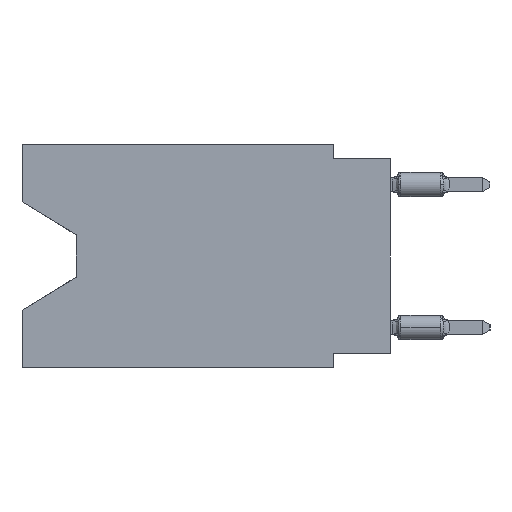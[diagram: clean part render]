
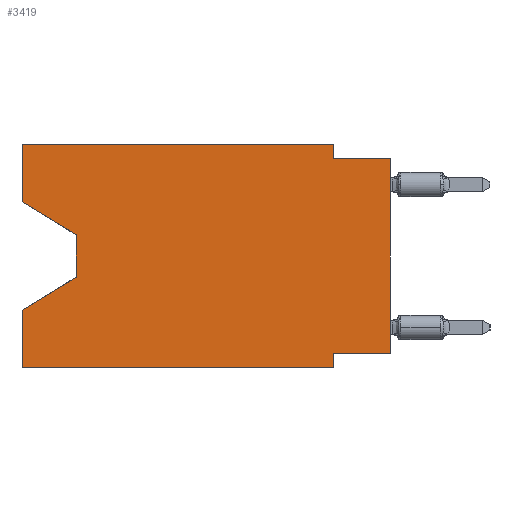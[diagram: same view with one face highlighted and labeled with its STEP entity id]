
A CAD part, left-side view. The second image highlights one B-rep face of the part: STEP entity #3419.
In plain terms, the highlighted planar face has unit normal (-1, 0, 0).
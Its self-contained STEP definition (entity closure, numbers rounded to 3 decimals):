
#75 = CARTESIAN_POINT ( 'NONE',  ( 0., 16.383, 0. ) ) ;
#409 = VERTEX_POINT ( 'NONE', #22014 ) ;
#544 = LINE ( 'NONE', #12322, #35364 ) ;
#1383 = DIRECTION ( 'NONE',  ( 0., -0.855, -0.519 ) ) ;
#1405 = ORIENTED_EDGE ( 'NONE', *, *, #28028, .F. ) ;
#1562 = DIRECTION ( 'NONE',  ( 0., 0., -1. ) ) ;
#2207 = DIRECTION ( 'NONE',  ( 0., 0.855, -0.519 ) ) ;
#2559 = VECTOR ( 'NONE', #2207, 1000. ) ;
#2894 = DIRECTION ( 'NONE',  ( 0., 0., -1. ) ) ;
#3386 = CARTESIAN_POINT ( 'NONE',  ( 0., 0., -9.271 ) ) ;
#3419 = ADVANCED_FACE ( 'NONE', ( #14137 ), #25959, .F. ) ;
#3909 = VERTEX_POINT ( 'NONE', #11076 ) ;
#5049 = EDGE_CURVE ( 'NONE', #409, #8129, #7990, .T. ) ;
#5308 = CARTESIAN_POINT ( 'NONE',  ( 0., 13.97, -5.893 ) ) ;
#6658 = CARTESIAN_POINT ( 'NONE',  ( 0., 16.383, -9.906 ) ) ;
#6813 = LINE ( 'NONE', #12984, #12689 ) ;
#7550 = CARTESIAN_POINT ( 'NONE',  ( 0., 2.54, -0.635 ) ) ;
#7679 = CARTESIAN_POINT ( 'NONE',  ( 0., 16.383, -2.546 ) ) ;
#7990 = LINE ( 'NONE', #5308, #2559 ) ;
#8129 = VERTEX_POINT ( 'NONE', #30926 ) ;
#8517 = EDGE_CURVE ( 'NONE', #10691, #29072, #544, .T. ) ;
#8570 = LINE ( 'NONE', #75, #35928 ) ;
#8912 = DIRECTION ( 'NONE',  ( 1., 0., 0. ) ) ;
#9150 = DIRECTION ( 'NONE',  ( 0., 0., 1. ) ) ;
#9357 = DIRECTION ( 'NONE',  ( 0., 1., 0. ) ) ;
#9603 = VECTOR ( 'NONE', #15794, 1000. ) ;
#9786 = VECTOR ( 'NONE', #32987, 1000. ) ;
#10060 = ORIENTED_EDGE ( 'NONE', *, *, #29583, .T. ) ;
#10117 = VECTOR ( 'NONE', #2894, 1000. ) ;
#10691 = VERTEX_POINT ( 'NONE', #7550 ) ;
#11076 = CARTESIAN_POINT ( 'NONE',  ( 0., 2.54, -9.271 ) ) ;
#12077 = LINE ( 'NONE', #3386, #18092 ) ;
#12322 = CARTESIAN_POINT ( 'NONE',  ( 0., 0., -0.635 ) ) ;
#12349 = CARTESIAN_POINT ( 'NONE',  ( 0., 16.383, 0. ) ) ;
#12626 = EDGE_CURVE ( 'NONE', #19016, #3909, #12077, .T. ) ;
#12689 = VECTOR ( 'NONE', #1383, 1000. ) ;
#12698 = LINE ( 'NONE', #18308, #9603 ) ;
#12715 = EDGE_CURVE ( 'NONE', #28179, #22189, #30252, .T. ) ;
#12984 = CARTESIAN_POINT ( 'NONE',  ( 0., 16.383, -2.546 ) ) ;
#13212 = ORIENTED_EDGE ( 'NONE', *, *, #19377, .T. ) ;
#14137 = FACE_OUTER_BOUND ( 'NONE', #32983, .T. ) ;
#14534 = ORIENTED_EDGE ( 'NONE', *, *, #25354, .F. ) ;
#14925 = LINE ( 'NONE', #23454, #29305 ) ;
#15179 = DIRECTION ( 'NONE',  ( 0., 0., 1. ) ) ;
#15706 = VECTOR ( 'NONE', #21638, 1000. ) ;
#15775 = CARTESIAN_POINT ( 'NONE',  ( 0., 16.383, -9.906 ) ) ;
#15794 = DIRECTION ( 'NONE',  ( 0., 0., 1. ) ) ;
#16940 = ORIENTED_EDGE ( 'NONE', *, *, #20787, .T. ) ;
#17511 = EDGE_CURVE ( 'NONE', #36996, #10691, #26676, .T. ) ;
#18067 = CARTESIAN_POINT ( 'NONE',  ( 0., 16.383, 0. ) ) ;
#18092 = VECTOR ( 'NONE', #9357, 1000. ) ;
#18308 = CARTESIAN_POINT ( 'NONE',  ( 0., 0., 0. ) ) ;
#18381 = EDGE_CURVE ( 'NONE', #3909, #23698, #22638, .T. ) ;
#19016 = VERTEX_POINT ( 'NONE', #21206 ) ;
#19377 = EDGE_CURVE ( 'NONE', #23972, #409, #14925, .T. ) ;
#20613 = ORIENTED_EDGE ( 'NONE', *, *, #12626, .F. ) ;
#20787 = EDGE_CURVE ( 'NONE', #28179, #23972, #6813, .T. ) ;
#20856 = ORIENTED_EDGE ( 'NONE', *, *, #18381, .F. ) ;
#21206 = CARTESIAN_POINT ( 'NONE',  ( 0., 0., -9.271 ) ) ;
#21638 = DIRECTION ( 'NONE',  ( 0., -1., 0. ) ) ;
#22014 = CARTESIAN_POINT ( 'NONE',  ( 0., 13.97, -5.893 ) ) ;
#22189 = VERTEX_POINT ( 'NONE', #12349 ) ;
#22638 = LINE ( 'NONE', #34410, #29856 ) ;
#22715 = CARTESIAN_POINT ( 'NONE',  ( 0., 2.54, 0. ) ) ;
#23079 = VERTEX_POINT ( 'NONE', #6658 ) ;
#23454 = CARTESIAN_POINT ( 'NONE',  ( 0., 13.97, -4.013 ) ) ;
#23698 = VERTEX_POINT ( 'NONE', #38198 ) ;
#23972 = VERTEX_POINT ( 'NONE', #36436 ) ;
#25354 = EDGE_CURVE ( 'NONE', #23079, #8129, #8570, .T. ) ;
#25959 = PLANE ( 'NONE',  #29307 ) ;
#26676 = LINE ( 'NONE', #29955, #10117 ) ;
#27044 = ORIENTED_EDGE ( 'NONE', *, *, #5049, .T. ) ;
#27396 = LINE ( 'NONE', #15775, #9786 ) ;
#27455 = LINE ( 'NONE', #33604, #15706 ) ;
#27547 = ORIENTED_EDGE ( 'NONE', *, *, #12715, .F. ) ;
#28028 = EDGE_CURVE ( 'NONE', #22189, #36996, #27455, .T. ) ;
#28179 = VERTEX_POINT ( 'NONE', #7679 ) ;
#29061 = DIRECTION ( 'NONE',  ( 0., 0., -1. ) ) ;
#29072 = VERTEX_POINT ( 'NONE', #35177 ) ;
#29305 = VECTOR ( 'NONE', #29061, 1000. ) ;
#29307 = AXIS2_PLACEMENT_3D ( 'NONE', #37931, #8912, #35400 ) ;
#29583 = EDGE_CURVE ( 'NONE', #19016, #29072, #12698, .T. ) ;
#29856 = VECTOR ( 'NONE', #1562, 1000. ) ;
#29955 = CARTESIAN_POINT ( 'NONE',  ( 0., 2.54, 0. ) ) ;
#30252 = LINE ( 'NONE', #18067, #37203 ) ;
#30926 = CARTESIAN_POINT ( 'NONE',  ( 0., 16.383, -7.36 ) ) ;
#32983 = EDGE_LOOP ( 'NONE', ( #16940, #13212, #27044, #14534, #35292, #20856, #20613, #10060, #37330, #33907, #1405, #27547 ) ) ;
#32987 = DIRECTION ( 'NONE',  ( 0., -1., 0. ) ) ;
#33604 = CARTESIAN_POINT ( 'NONE',  ( 0., 16.383, 0. ) ) ;
#33907 = ORIENTED_EDGE ( 'NONE', *, *, #17511, .F. ) ;
#34410 = CARTESIAN_POINT ( 'NONE',  ( 0., 2.54, -9.906 ) ) ;
#35177 = CARTESIAN_POINT ( 'NONE',  ( 0., 0., -0.635 ) ) ;
#35292 = ORIENTED_EDGE ( 'NONE', *, *, #36915, .T. ) ;
#35364 = VECTOR ( 'NONE', #35908, 1000. ) ;
#35400 = DIRECTION ( 'NONE',  ( 0., 0., -1. ) ) ;
#35908 = DIRECTION ( 'NONE',  ( 0., -1., 0. ) ) ;
#35928 = VECTOR ( 'NONE', #9150, 1000. ) ;
#36436 = CARTESIAN_POINT ( 'NONE',  ( 0., 13.97, -4.013 ) ) ;
#36915 = EDGE_CURVE ( 'NONE', #23079, #23698, #27396, .T. ) ;
#36996 = VERTEX_POINT ( 'NONE', #22715 ) ;
#37203 = VECTOR ( 'NONE', #15179, 1000. ) ;
#37330 = ORIENTED_EDGE ( 'NONE', *, *, #8517, .F. ) ;
#37931 = CARTESIAN_POINT ( 'NONE',  ( 0., 16.383, 0. ) ) ;
#38198 = CARTESIAN_POINT ( 'NONE',  ( 0., 2.54, -9.906 ) ) ;
